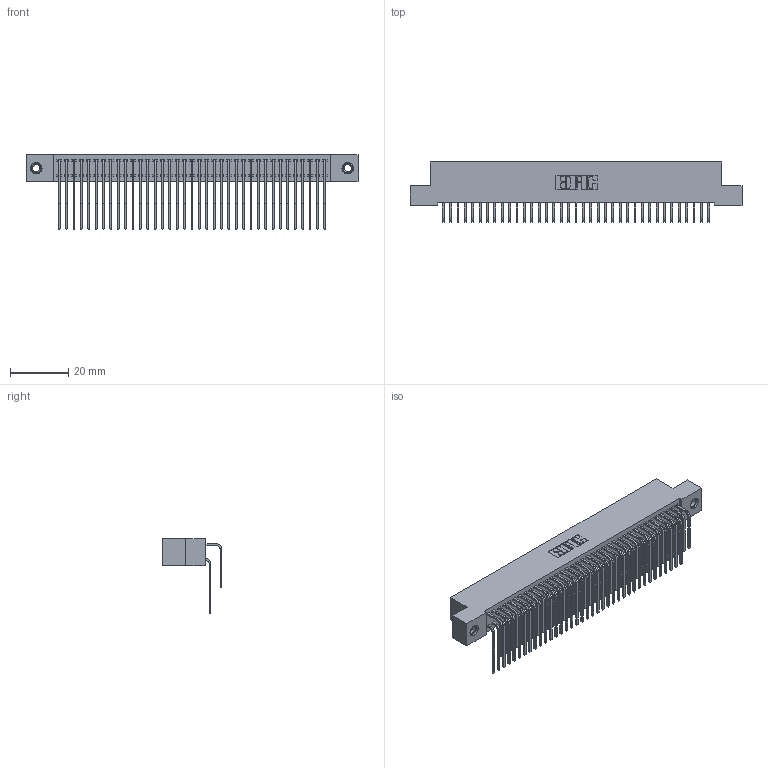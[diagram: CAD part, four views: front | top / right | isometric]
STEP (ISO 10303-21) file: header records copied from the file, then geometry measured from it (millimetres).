
FILE_DESCRIPTION (( 'STEP AP203' ), '1' );
FILE_NAME ('342-074-559-207.STEP', '2018-08-13T11:53:52', ( '' ), ( '' ), 'SwSTEP 2.0', 'SolidWorks 2016', '' );
FILE_SCHEMA (( 'CONFIG_CONTROL_DESIGN' ));
Length unit declared in the file: inch
Products named in the file (5): 345-250-001_345-250-005-103; 342-074-559-207; 342 Part_TI; 345-292-001_558 559 Tail - 1; 345-292-001_559 Tail - 2
Assembly tree (77 placements, depth 2):
  342-074-559-207
    342 Part_TI
    345-292-001_558 559 Tail - 1  x37
    345-292-001_559 Tail - 2  x37
    345-250-001_345-250-005-103  x2
Bounding box: 114.3 x 20.64 x 25.78 mm (x, y, z)
Volume: 10660.4 mm3; surface area: 19186.1 mm2
Topology: 77 solids, 77 shells, 4166 faces, 12349 edges, 8126 vertices
Faces by surface type: plane 2910, cylinder 1240, cone 12, torus 4
Entity records: 27288 total; most frequent: CARTESIAN_POINT 4560, ORIENTED_EDGE 4438, DIRECTION 3917, EDGE_CURVE 2219, LINE 2031, VECTOR 2031, VERTEX_POINT 1472, AXIS2_PLACEMENT_3D 943
